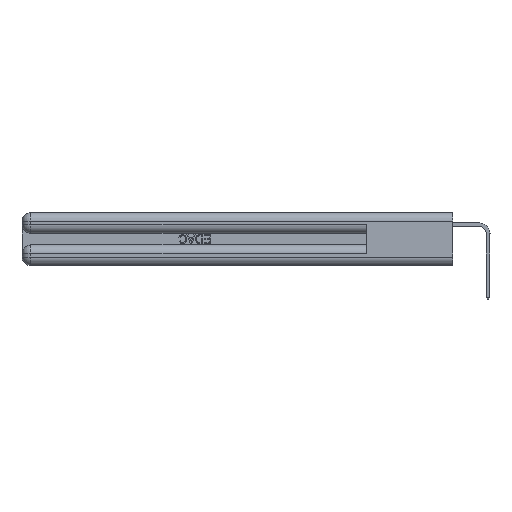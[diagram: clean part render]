
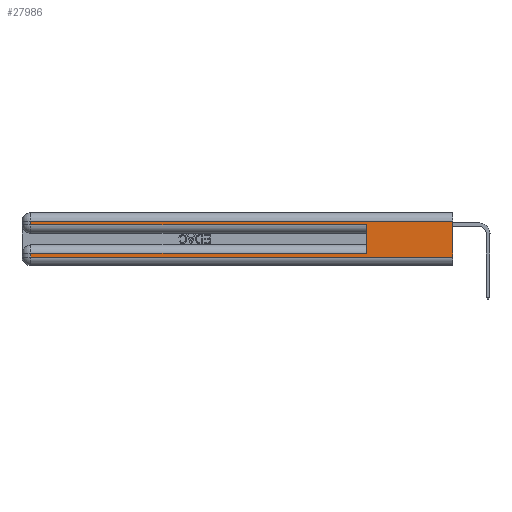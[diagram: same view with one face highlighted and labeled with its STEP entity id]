
A CAD part, left-side view. The second image highlights one B-rep face of the part: STEP entity #27986.
In plain terms, the highlighted planar face has unit normal (-1, 0, 0).
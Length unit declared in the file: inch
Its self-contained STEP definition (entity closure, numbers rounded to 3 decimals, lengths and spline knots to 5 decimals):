
#330 = VERTEX_POINT ( 'NONE', #41812 ) ;
#610 = EDGE_CURVE ( 'NONE', #43923, #25299, #18566, .T. ) ;
#1803 = VERTEX_POINT ( 'NONE', #10932 ) ;
#2466 = VERTEX_POINT ( 'NONE', #33366 ) ;
#4021 = CARTESIAN_POINT ( 'NONE',  ( 0., 0., 0.06 ) ) ;
#4431 = VECTOR ( 'NONE', #7524, 39.37008 ) ;
#4877 = DIRECTION ( 'NONE',  ( 0., 0., -1. ) ) ;
#5544 = PLANE ( 'NONE',  #36272 ) ;
#5735 = LINE ( 'NONE', #29925, #42422 ) ;
#6188 = FACE_OUTER_BOUND ( 'NONE', #40146, .T. ) ;
#6337 = CARTESIAN_POINT ( 'NONE',  ( 0., 0., 0.37 ) ) ;
#6620 = CARTESIAN_POINT ( 'NONE',  ( 0., 2.94, 0.285 ) ) ;
#7524 = DIRECTION ( 'NONE',  ( 0., 0., 1. ) ) ;
#9853 = VECTOR ( 'NONE', #33802, 39.37008 ) ;
#10932 = CARTESIAN_POINT ( 'NONE',  ( 0., 0.6, 0.285 ) ) ;
#11109 = CARTESIAN_POINT ( 'NONE',  ( 0., 0.6, 0.145 ) ) ;
#12015 = VECTOR ( 'NONE', #36996, 39.37008 ) ;
#12718 = CARTESIAN_POINT ( 'NONE',  ( 0., 0., 0.37 ) ) ;
#12965 = EDGE_CURVE ( 'NONE', #330, #2466, #40348, .T. ) ;
#15439 = ORIENTED_EDGE ( 'NONE', *, *, #30070, .T. ) ;
#16282 = DIRECTION ( 'NONE',  ( 1., 0., 0. ) ) ;
#16882 = ORIENTED_EDGE ( 'NONE', *, *, #29400, .F. ) ;
#17412 = LINE ( 'NONE', #29772, #36319 ) ;
#17650 = VECTOR ( 'NONE', #24781, 39.37008 ) ;
#18325 = EDGE_CURVE ( 'NONE', #29501, #28176, #17412, .T. ) ;
#18353 = CARTESIAN_POINT ( 'NONE',  ( 0., 0., 0.06 ) ) ;
#18397 = EDGE_CURVE ( 'NONE', #2466, #43923, #5735, .T. ) ;
#18566 = LINE ( 'NONE', #18353, #28012 ) ;
#18616 = ORIENTED_EDGE ( 'NONE', *, *, #18397, .T. ) ;
#20502 = VECTOR ( 'NONE', #38338, 39.37008 ) ;
#21205 = CARTESIAN_POINT ( 'NONE',  ( 0., 0., 0.31 ) ) ;
#21596 = CARTESIAN_POINT ( 'NONE',  ( 0., 2.94, 0.06 ) ) ;
#21914 = DIRECTION ( 'NONE',  ( 0., -1., 0. ) ) ;
#23230 = DIRECTION ( 'NONE',  ( 0., 0., -1. ) ) ;
#24781 = DIRECTION ( 'NONE',  ( 0., 1., 0. ) ) ;
#25299 = VERTEX_POINT ( 'NONE', #4021 ) ;
#26307 = CARTESIAN_POINT ( 'NONE',  ( 0., 0., 0.085 ) ) ;
#26475 = ORIENTED_EDGE ( 'NONE', *, *, #38710, .F. ) ;
#27109 = LINE ( 'NONE', #21205, #17650 ) ;
#27661 = LINE ( 'NONE', #44555, #9853 ) ;
#27772 = ORIENTED_EDGE ( 'NONE', *, *, #40430, .T. ) ;
#27986 = ADVANCED_FACE ( 'NONE', ( #6188 ), #5544, .F. ) ;
#28012 = VECTOR ( 'NONE', #21914, 39.37008 ) ;
#28176 = VERTEX_POINT ( 'NONE', #6620 ) ;
#28397 = CARTESIAN_POINT ( 'NONE',  ( 0., 2.94, 0.31 ) ) ;
#28841 = VERTEX_POINT ( 'NONE', #32002 ) ;
#29400 = EDGE_CURVE ( 'NONE', #28841, #25299, #31064, .T. ) ;
#29501 = VERTEX_POINT ( 'NONE', #28397 ) ;
#29772 = CARTESIAN_POINT ( 'NONE',  ( 0., 2.94, 0.37 ) ) ;
#29821 = ORIENTED_EDGE ( 'NONE', *, *, #610, .T. ) ;
#29925 = CARTESIAN_POINT ( 'NONE',  ( 0., 2.94, 0.37 ) ) ;
#30070 = EDGE_CURVE ( 'NONE', #28841, #29501, #27109, .T. ) ;
#31064 = LINE ( 'NONE', #6337, #20502 ) ;
#32002 = CARTESIAN_POINT ( 'NONE',  ( 0., 0., 0.31 ) ) ;
#32781 = LINE ( 'NONE', #11109, #4431 ) ;
#33366 = CARTESIAN_POINT ( 'NONE',  ( 0., 2.94, 0.085 ) ) ;
#33802 = DIRECTION ( 'NONE',  ( 0., -1., 0. ) ) ;
#36272 = AXIS2_PLACEMENT_3D ( 'NONE', #12718, #16282, #41152 ) ;
#36319 = VECTOR ( 'NONE', #4877, 39.37008 ) ;
#36996 = DIRECTION ( 'NONE',  ( 0., 1., 0. ) ) ;
#37686 = ORIENTED_EDGE ( 'NONE', *, *, #12965, .T. ) ;
#38059 = ORIENTED_EDGE ( 'NONE', *, *, #18325, .T. ) ;
#38338 = DIRECTION ( 'NONE',  ( 0., 0., -1. ) ) ;
#38710 = EDGE_CURVE ( 'NONE', #330, #1803, #32781, .T. ) ;
#40146 = EDGE_LOOP ( 'NONE', ( #16882, #15439, #38059, #27772, #26475, #37686, #18616, #29821 ) ) ;
#40348 = LINE ( 'NONE', #26307, #12015 ) ;
#40430 = EDGE_CURVE ( 'NONE', #28176, #1803, #27661, .T. ) ;
#41152 = DIRECTION ( 'NONE',  ( 0., 0., -1. ) ) ;
#41812 = CARTESIAN_POINT ( 'NONE',  ( 0., 0.6, 0.085 ) ) ;
#42422 = VECTOR ( 'NONE', #23230, 39.37008 ) ;
#43923 = VERTEX_POINT ( 'NONE', #21596 ) ;
#44555 = CARTESIAN_POINT ( 'NONE',  ( 0., 0., 0.285 ) ) ;
